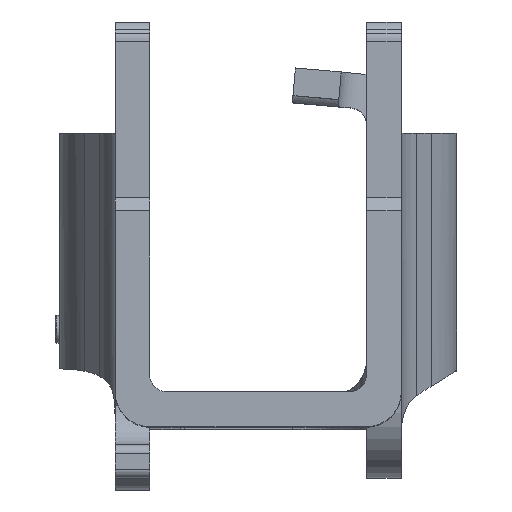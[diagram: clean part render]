
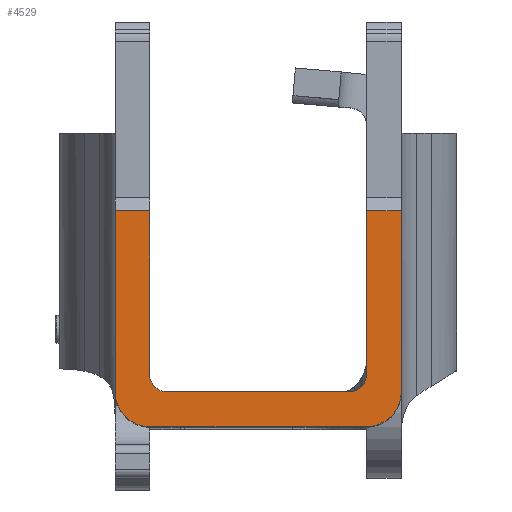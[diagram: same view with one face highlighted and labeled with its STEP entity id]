
A CAD part, top view. The second image highlights one B-rep face of the part: STEP entity #4529.
In plain terms, the highlighted planar face has unit normal (0, 0, 1).
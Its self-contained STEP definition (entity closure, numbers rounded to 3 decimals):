
#212=PLANE('',#4984);
#440=FACE_OUTER_BOUND('',#678,.T.);
#678=EDGE_LOOP('',(#4185,#4186,#4187,#4188,#4189,#4190,#4191,#4192,#4193,
#4194,#4195,#4196));
#704=LINE('',#6397,#1143);
#724=LINE('',#6460,#1163);
#736=LINE('',#6487,#1175);
#751=LINE('',#6532,#1190);
#1010=LINE('',#7513,#1449);
#1011=LINE('',#7515,#1450);
#1035=LINE('',#7611,#1474);
#1079=LINE('',#7748,#1518);
#1143=VECTOR('',#5058,10.);
#1163=VECTOR('',#5110,10.);
#1175=VECTOR('',#5134,10.);
#1190=VECTOR('',#5169,10.);
#1449=VECTOR('',#5936,10.);
#1450=VECTOR('',#5939,10.);
#1474=VECTOR('',#6023,10.);
#1518=VECTOR('',#6175,10.);
#1722=CIRCLE('',#4921,1.);
#1723=CIRCLE('',#4928,2.);
#1724=CIRCLE('',#4936,2.);
#1726=CIRCLE('',#4940,1.);
#1765=VERTEX_POINT('',#6394);
#1766=VERTEX_POINT('',#6396);
#1792=VERTEX_POINT('',#6457);
#1793=VERTEX_POINT('',#6459);
#1801=VERTEX_POINT('',#6484);
#1802=VERTEX_POINT('',#6486);
#1821=VERTEX_POINT('',#6529);
#1822=VERTEX_POINT('',#6531);
#2148=VERTEX_POINT('',#7607);
#2150=VERTEX_POINT('',#7610);
#2172=VERTEX_POINT('',#7720);
#2173=VERTEX_POINT('',#7744);
#2216=EDGE_CURVE('',#1766,#1765,#704,.T.);
#2247=EDGE_CURVE('',#1793,#1792,#724,.T.);
#2261=EDGE_CURVE('',#1802,#1801,#736,.T.);
#2284=EDGE_CURVE('',#1822,#1821,#751,.T.);
#2705=EDGE_CURVE('',#1801,#1793,#1010,.T.);
#2706=EDGE_CURVE('',#1821,#1766,#1011,.T.);
#2744=EDGE_CURVE('',#2150,#2148,#1035,.T.);
#2795=EDGE_CURVE('',#2150,#1765,#1722,.T.);
#2800=EDGE_CURVE('',#2172,#1792,#1723,.T.);
#2805=EDGE_CURVE('',#1822,#2173,#1724,.T.);
#2807=EDGE_CURVE('',#2172,#2173,#1079,.T.);
#2809=EDGE_CURVE('',#1802,#2148,#1726,.T.);
#4185=ORIENTED_EDGE('',*,*,#2706,.T.);
#4186=ORIENTED_EDGE('',*,*,#2216,.T.);
#4187=ORIENTED_EDGE('',*,*,#2795,.F.);
#4188=ORIENTED_EDGE('',*,*,#2744,.T.);
#4189=ORIENTED_EDGE('',*,*,#2809,.F.);
#4190=ORIENTED_EDGE('',*,*,#2261,.T.);
#4191=ORIENTED_EDGE('',*,*,#2705,.T.);
#4192=ORIENTED_EDGE('',*,*,#2247,.T.);
#4193=ORIENTED_EDGE('',*,*,#2800,.F.);
#4194=ORIENTED_EDGE('',*,*,#2807,.T.);
#4195=ORIENTED_EDGE('',*,*,#2805,.F.);
#4196=ORIENTED_EDGE('',*,*,#2284,.T.);
#4529=ADVANCED_FACE('',(#440),#212,.T.);
#4921=AXIS2_PLACEMENT_3D('',#7710,#6134,#6135);
#4928=AXIS2_PLACEMENT_3D('',#7722,#6152,#6153);
#4936=AXIS2_PLACEMENT_3D('',#7745,#6170,#6171);
#4940=AXIS2_PLACEMENT_3D('',#7752,#6180,#6181);
#4984=AXIS2_PLACEMENT_3D('',#7834,#6306,#6307);
#5058=DIRECTION('',(0.,-1.,0.));
#5110=DIRECTION('',(0.,-1.,0.));
#5134=DIRECTION('',(0.,1.,0.));
#5169=DIRECTION('',(0.,1.,0.));
#5936=DIRECTION('',(-1.,0.,0.));
#5939=DIRECTION('',(-1.,0.,0.));
#6023=DIRECTION('',(-1.,0.,0.));
#6134=DIRECTION('center_axis',(0.,0.,1.));
#6135=DIRECTION('ref_axis',(0.707,-0.707,0.));
#6152=DIRECTION('center_axis',(0.,0.,-1.));
#6153=DIRECTION('ref_axis',(-0.707,-0.707,0.));
#6170=DIRECTION('center_axis',(0.,0.,-1.));
#6171=DIRECTION('ref_axis',(0.707,-0.707,0.));
#6175=DIRECTION('',(1.,0.,0.));
#6180=DIRECTION('center_axis',(0.,0.,1.));
#6181=DIRECTION('ref_axis',(-0.707,-0.707,0.));
#6306=DIRECTION('center_axis',(0.,0.,1.));
#6307=DIRECTION('ref_axis',(1.,0.,0.));
#6394=CARTESIAN_POINT('',(6.25,-15.8,110.25));
#6396=CARTESIAN_POINT('',(6.25,-6.36,110.25));
#6397=CARTESIAN_POINT('',(6.25,-1.81,110.25));
#6457=CARTESIAN_POINT('',(-8.25,-16.8,110.25));
#6459=CARTESIAN_POINT('',(-8.25,-6.36,110.25));
#6460=CARTESIAN_POINT('',(-8.25,-1.81,110.25));
#6484=CARTESIAN_POINT('',(-6.25,-6.36,110.25));
#6486=CARTESIAN_POINT('',(-6.25,-15.8,110.25));
#6487=CARTESIAN_POINT('',(-6.25,-16.8,110.25));
#6529=CARTESIAN_POINT('',(8.25,-6.36,110.25));
#6531=CARTESIAN_POINT('',(8.25,-16.8,110.25));
#6532=CARTESIAN_POINT('',(8.25,-18.8,110.25));
#7513=CARTESIAN_POINT('',(4.125,-6.36,110.25));
#7515=CARTESIAN_POINT('',(4.125,-6.36,110.25));
#7607=CARTESIAN_POINT('',(-5.25,-16.8,110.25));
#7610=CARTESIAN_POINT('',(5.25,-16.8,110.25));
#7611=CARTESIAN_POINT('',(6.25,-16.8,110.25));
#7710=CARTESIAN_POINT('Origin',(5.25,-15.8,110.25));
#7720=CARTESIAN_POINT('',(-6.25,-18.8,110.25));
#7722=CARTESIAN_POINT('Origin',(-6.25,-16.8,110.25));
#7744=CARTESIAN_POINT('',(6.25,-18.8,110.25));
#7745=CARTESIAN_POINT('Origin',(6.25,-16.8,110.25));
#7748=CARTESIAN_POINT('',(-8.25,-18.8,110.25));
#7752=CARTESIAN_POINT('Origin',(-5.25,-15.8,110.25));
#7834=CARTESIAN_POINT('Origin',(0.,-10.305,110.25));
